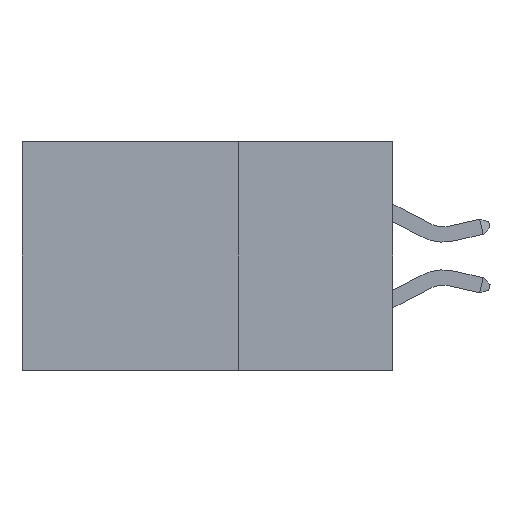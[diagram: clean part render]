
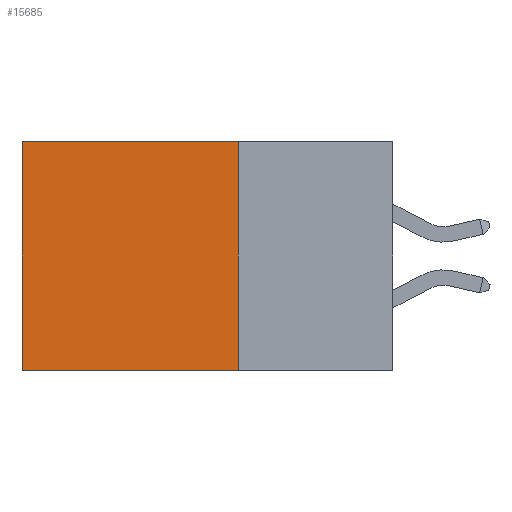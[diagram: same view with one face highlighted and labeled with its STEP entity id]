
A CAD part, left-side view. The second image highlights one B-rep face of the part: STEP entity #15685.
In plain terms, the highlighted planar face has unit normal (-1, 0, 0).
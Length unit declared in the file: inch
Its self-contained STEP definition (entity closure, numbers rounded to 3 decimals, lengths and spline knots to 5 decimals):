
#199 = EDGE_CURVE ( 'NONE', #11586, #12764, #12117, .T. ) ;
#1194 = ORIENTED_EDGE ( 'NONE', *, *, #39249, .T. ) ;
#1274 = VECTOR ( 'NONE', #7276, 39.37008 ) ;
#3399 = VERTEX_POINT ( 'NONE', #25835 ) ;
#7004 = ORIENTED_EDGE ( 'NONE', *, *, #27402, .F. ) ;
#7276 = DIRECTION ( 'NONE',  ( 0., 0., -1. ) ) ;
#11586 = VERTEX_POINT ( 'NONE', #28259 ) ;
#12117 = LINE ( 'NONE', #39780, #31090 ) ;
#12764 = VERTEX_POINT ( 'NONE', #28645 ) ;
#14904 = VERTEX_POINT ( 'NONE', #16919 ) ;
#15685 = ADVANCED_FACE ( 'NONE', ( #22639 ), #27767, .F. ) ;
#16202 = ORIENTED_EDGE ( 'NONE', *, *, #199, .T. ) ;
#16919 = CARTESIAN_POINT ( 'NONE',  ( 0.2875, 0.25, -0.37 ) ) ;
#17202 = CARTESIAN_POINT ( 'NONE',  ( 0.2875, 0.25, 0. ) ) ;
#17742 = CARTESIAN_POINT ( 'NONE',  ( 0.2875, 0.25, 0. ) ) ;
#18194 = DIRECTION ( 'NONE',  ( 1., 0., 0. ) ) ;
#22639 = FACE_OUTER_BOUND ( 'NONE', #32519, .T. ) ;
#24417 = LINE ( 'NONE', #34452, #39694 ) ;
#25123 = EDGE_CURVE ( 'NONE', #3399, #14904, #33317, .T. ) ;
#25835 = CARTESIAN_POINT ( 'NONE',  ( 0.2875, 0.25, 0. ) ) ;
#27402 = EDGE_CURVE ( 'NONE', #14904, #12764, #41516, .T. ) ;
#27767 = PLANE ( 'NONE',  #39035 ) ;
#28259 = CARTESIAN_POINT ( 'NONE',  ( 0.2875, 0.6, 0. ) ) ;
#28645 = CARTESIAN_POINT ( 'NONE',  ( 0.2875, 0.6, -0.37 ) ) ;
#28896 = DIRECTION ( 'NONE',  ( 0., 1., 0. ) ) ;
#30024 = CARTESIAN_POINT ( 'NONE',  ( 0.2875, 0.25, -0.37 ) ) ;
#31090 = VECTOR ( 'NONE', #33897, 39.37008 ) ;
#32519 = EDGE_LOOP ( 'NONE', ( #16202, #7004, #36832, #1194 ) ) ;
#33317 = LINE ( 'NONE', #17202, #1274 ) ;
#33897 = DIRECTION ( 'NONE',  ( 0., 0., -1. ) ) ;
#34452 = CARTESIAN_POINT ( 'NONE',  ( 0.2875, 0.25, 0. ) ) ;
#36832 = ORIENTED_EDGE ( 'NONE', *, *, #25123, .F. ) ;
#39035 = AXIS2_PLACEMENT_3D ( 'NONE', #17742, #18194, #41271 ) ;
#39249 = EDGE_CURVE ( 'NONE', #3399, #11586, #24417, .T. ) ;
#39694 = VECTOR ( 'NONE', #28896, 39.37008 ) ;
#39780 = CARTESIAN_POINT ( 'NONE',  ( 0.2875, 0.6, 0. ) ) ;
#39890 = VECTOR ( 'NONE', #40411, 39.37008 ) ;
#40411 = DIRECTION ( 'NONE',  ( 0., 1., 0. ) ) ;
#41271 = DIRECTION ( 'NONE',  ( 0., 0., -1. ) ) ;
#41516 = LINE ( 'NONE', #30024, #39890 ) ;
